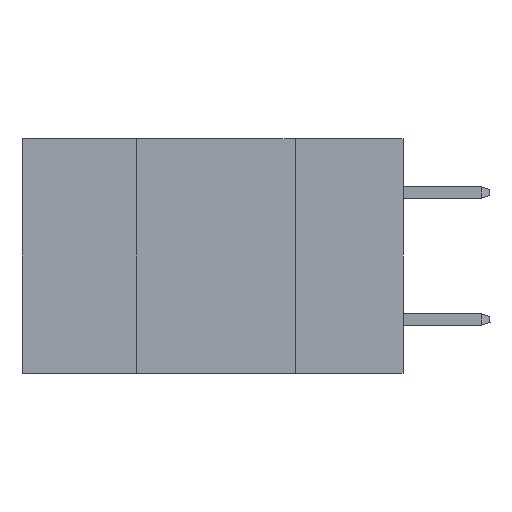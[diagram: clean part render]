
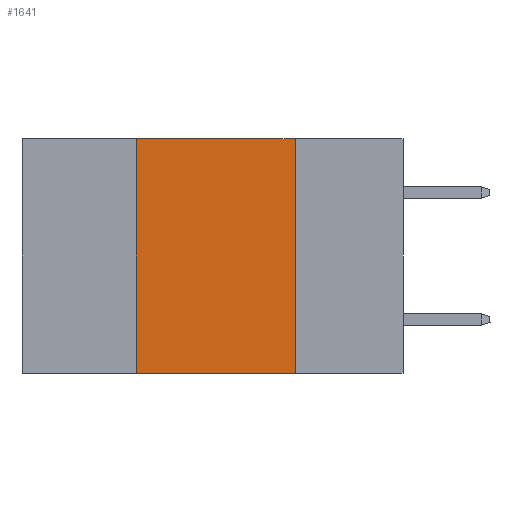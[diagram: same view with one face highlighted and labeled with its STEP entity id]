
A CAD part, left-side view. The second image highlights one B-rep face of the part: STEP entity #1641.
In plain terms, the highlighted planar face has unit normal (-1, 0, 0).
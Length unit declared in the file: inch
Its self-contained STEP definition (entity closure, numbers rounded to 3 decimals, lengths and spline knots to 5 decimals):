
#531 = CARTESIAN_POINT ( 'NONE',  ( 0., 0.42, -0.37 ) ) ;
#601 = VECTOR ( 'NONE', #13713, 39.37008 ) ;
#681 = VECTOR ( 'NONE', #4666, 39.37008 ) ;
#871 = AXIS2_PLACEMENT_3D ( 'NONE', #19943, #18244, #1663 ) ;
#1519 = ORIENTED_EDGE ( 'NONE', *, *, #12107, .F. ) ;
#1641 = ADVANCED_FACE ( 'NONE', ( #5237 ), #13368, .F. ) ;
#1663 = DIRECTION ( 'NONE',  ( 0., 0., -1. ) ) ;
#3628 = LINE ( 'NONE', #3852, #601 ) ;
#3852 = CARTESIAN_POINT ( 'NONE',  ( 0., 0.42, 0. ) ) ;
#3870 = LINE ( 'NONE', #13508, #12328 ) ;
#4355 = EDGE_LOOP ( 'NONE', ( #10809, #4636, #1519, #9589 ) ) ;
#4636 = ORIENTED_EDGE ( 'NONE', *, *, #16272, .F. ) ;
#4666 = DIRECTION ( 'NONE',  ( 0., -1., 0. ) ) ;
#5237 = FACE_OUTER_BOUND ( 'NONE', #4355, .T. ) ;
#6336 = VERTEX_POINT ( 'NONE', #19262 ) ;
#8810 = VERTEX_POINT ( 'NONE', #531 ) ;
#9589 = ORIENTED_EDGE ( 'NONE', *, *, #15974, .T. ) ;
#10616 = EDGE_CURVE ( 'NONE', #14831, #6336, #3870, .T. ) ;
#10809 = ORIENTED_EDGE ( 'NONE', *, *, #10616, .F. ) ;
#11175 = LINE ( 'NONE', #17787, #681 ) ;
#12107 = EDGE_CURVE ( 'NONE', #8810, #16252, #3628, .T. ) ;
#12328 = VECTOR ( 'NONE', #20306, 39.37008 ) ;
#12462 = CARTESIAN_POINT ( 'NONE',  ( 0., 0.42, 0. ) ) ;
#12755 = CARTESIAN_POINT ( 'NONE',  ( 0., 0.17, 0. ) ) ;
#13368 = PLANE ( 'NONE',  #871 ) ;
#13508 = CARTESIAN_POINT ( 'NONE',  ( 0., 0.17, 0. ) ) ;
#13713 = DIRECTION ( 'NONE',  ( 0., 0., 1. ) ) ;
#13883 = CARTESIAN_POINT ( 'NONE',  ( 0., 0.6, 0. ) ) ;
#14831 = VERTEX_POINT ( 'NONE', #12755 ) ;
#15974 = EDGE_CURVE ( 'NONE', #8810, #6336, #11175, .T. ) ;
#16252 = VERTEX_POINT ( 'NONE', #12462 ) ;
#16272 = EDGE_CURVE ( 'NONE', #16252, #14831, #17451, .T. ) ;
#17451 = LINE ( 'NONE', #13883, #17628 ) ;
#17628 = VECTOR ( 'NONE', #20658, 39.37008 ) ;
#17787 = CARTESIAN_POINT ( 'NONE',  ( 0., 0.6, -0.37 ) ) ;
#18244 = DIRECTION ( 'NONE',  ( 1., 0., 0. ) ) ;
#19262 = CARTESIAN_POINT ( 'NONE',  ( 0., 0.17, -0.37 ) ) ;
#19943 = CARTESIAN_POINT ( 'NONE',  ( 0., 0.6, 0. ) ) ;
#20306 = DIRECTION ( 'NONE',  ( 0., 0., -1. ) ) ;
#20658 = DIRECTION ( 'NONE',  ( 0., -1., 0. ) ) ;
